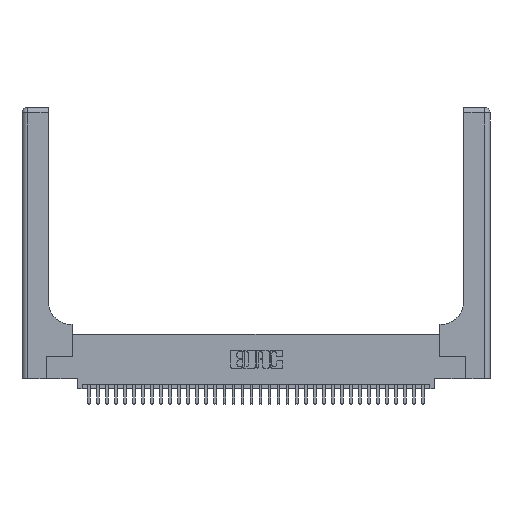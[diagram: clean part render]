
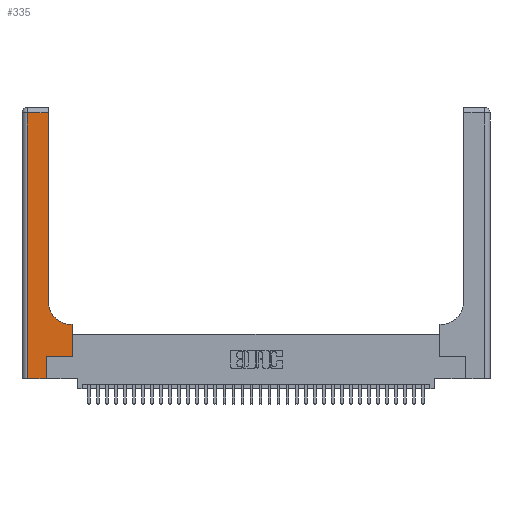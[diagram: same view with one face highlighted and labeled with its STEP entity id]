
A CAD part, top view. The second image highlights one B-rep face of the part: STEP entity #335.
In plain terms, the highlighted planar face has unit normal (0, 0, 1).
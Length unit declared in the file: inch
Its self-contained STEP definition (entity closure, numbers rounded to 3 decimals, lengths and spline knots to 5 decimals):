
#335 = ADVANCED_FACE ( 'NONE', ( #9375 ), #31112, .F. ) ;
#1353 = CARTESIAN_POINT ( 'NONE',  ( 0.269, 0.25, 0.37 ) ) ;
#1536 = DIRECTION ( 'NONE',  ( 0., 1., 0. ) ) ;
#1728 = VECTOR ( 'NONE', #20015, 39.37008 ) ;
#2449 = EDGE_CURVE ( 'NONE', #31710, #33358, #18399, .T. ) ;
#2634 = VECTOR ( 'NONE', #32224, 39.37008 ) ;
#2716 = AXIS2_PLACEMENT_3D ( 'NONE', #5078, #10599, #8089 ) ;
#4294 = DIRECTION ( 'NONE',  ( -1., 0., 0. ) ) ;
#4831 = DIRECTION ( 'NONE',  ( 1., 0., 0. ) ) ;
#5078 = CARTESIAN_POINT ( 'NONE',  ( 0.5415, 0.85, 0.37 ) ) ;
#5316 = CARTESIAN_POINT ( 'NONE',  ( 0.2915, 0.85, 0.37 ) ) ;
#5920 = LINE ( 'NONE', #24273, #15427 ) ;
#6356 = EDGE_CURVE ( 'NONE', #29898, #30478, #5920, .T. ) ;
#7204 = DIRECTION ( 'NONE',  ( 0., 0., -1. ) ) ;
#7318 = DIRECTION ( 'NONE',  ( -1., 0., 0. ) ) ;
#7488 = CARTESIAN_POINT ( 'NONE',  ( 0.269, 0.25, 0.37 ) ) ;
#8022 = CARTESIAN_POINT ( 'NONE',  ( 0.5585, 0.6, 0.37 ) ) ;
#8089 = DIRECTION ( 'NONE',  ( 1., 0., 0. ) ) ;
#8786 = AXIS2_PLACEMENT_3D ( 'NONE', #29046, #7204, #7318 ) ;
#9375 = FACE_OUTER_BOUND ( 'NONE', #27421, .T. ) ;
#10599 = DIRECTION ( 'NONE',  ( 0., 0., -1. ) ) ;
#10969 = EDGE_CURVE ( 'NONE', #17357, #12813, #31996, .T. ) ;
#10972 = DIRECTION ( 'NONE',  ( 0., 1., 0. ) ) ;
#11022 = VECTOR ( 'NONE', #26573, 39.37008 ) ;
#11787 = EDGE_CURVE ( 'NONE', #12813, #29898, #18621, .T. ) ;
#12808 = DIRECTION ( 'NONE',  ( 0., 1., 0. ) ) ;
#12813 = VERTEX_POINT ( 'NONE', #34967 ) ;
#13652 = LINE ( 'NONE', #15150, #22717 ) ;
#13897 = EDGE_CURVE ( 'NONE', #25910, #35000, #18821, .T. ) ;
#14307 = ORIENTED_EDGE ( 'NONE', *, *, #10969, .T. ) ;
#15150 = CARTESIAN_POINT ( 'NONE',  ( 0., 2.94, 0.37 ) ) ;
#15427 = VECTOR ( 'NONE', #12808, 39.37008 ) ;
#16515 = CARTESIAN_POINT ( 'NONE',  ( 0.06, 2.94, 0.37 ) ) ;
#17136 = LINE ( 'NONE', #7488, #26599 ) ;
#17357 = VERTEX_POINT ( 'NONE', #16515 ) ;
#18399 = LINE ( 'NONE', #34690, #11022 ) ;
#18621 = LINE ( 'NONE', #26267, #2634 ) ;
#18821 = LINE ( 'NONE', #30571, #29158 ) ;
#19209 = CARTESIAN_POINT ( 'NONE',  ( 0.5585, 0.25, 0.37 ) ) ;
#20015 = DIRECTION ( 'NONE',  ( 0., -1., 0. ) ) ;
#20751 = ORIENTED_EDGE ( 'NONE', *, *, #11787, .T. ) ;
#21375 = CARTESIAN_POINT ( 'NONE',  ( 0.5585, 0.25, 0.37 ) ) ;
#21390 = ORIENTED_EDGE ( 'NONE', *, *, #2449, .T. ) ;
#21697 = EDGE_CURVE ( 'NONE', #30478, #21902, #17136, .T. ) ;
#21788 = EDGE_CURVE ( 'NONE', #33358, #25910, #29222, .T. ) ;
#21902 = VERTEX_POINT ( 'NONE', #19209 ) ;
#22717 = VECTOR ( 'NONE', #4294, 39.37008 ) ;
#23096 = LINE ( 'NONE', #21375, #30869 ) ;
#23734 = CARTESIAN_POINT ( 'NONE',  ( 0.5415, 0.6, 0.37 ) ) ;
#24273 = CARTESIAN_POINT ( 'NONE',  ( 0.269, 0., 0.37 ) ) ;
#24621 = ORIENTED_EDGE ( 'NONE', *, *, #21697, .T. ) ;
#24869 = ORIENTED_EDGE ( 'NONE', *, *, #13897, .T. ) ;
#25910 = VERTEX_POINT ( 'NONE', #5316 ) ;
#26267 = CARTESIAN_POINT ( 'NONE',  ( 0., 0., 0.37 ) ) ;
#26573 = DIRECTION ( 'NONE',  ( -1., 0., 0. ) ) ;
#26599 = VECTOR ( 'NONE', #4831, 39.37008 ) ;
#27421 = EDGE_LOOP ( 'NONE', ( #24869, #27992, #14307, #20751, #32278, #24621, #33480, #21390, #33287 ) ) ;
#27992 = ORIENTED_EDGE ( 'NONE', *, *, #30461, .T. ) ;
#29046 = CARTESIAN_POINT ( 'NONE',  ( 0., 3., 0.37 ) ) ;
#29158 = VECTOR ( 'NONE', #10972, 39.37008 ) ;
#29222 = CIRCLE ( 'NONE', #2716, 0.25 ) ;
#29898 = VERTEX_POINT ( 'NONE', #34853 ) ;
#30461 = EDGE_CURVE ( 'NONE', #35000, #17357, #13652, .T. ) ;
#30478 = VERTEX_POINT ( 'NONE', #1353 ) ;
#30571 = CARTESIAN_POINT ( 'NONE',  ( 0.2915, 3., 0.37 ) ) ;
#30867 = CARTESIAN_POINT ( 'NONE',  ( 0.06, 3., 0.37 ) ) ;
#30869 = VECTOR ( 'NONE', #1536, 39.37008 ) ;
#31112 = PLANE ( 'NONE',  #8786 ) ;
#31168 = CARTESIAN_POINT ( 'NONE',  ( 0.2915, 2.94, 0.37 ) ) ;
#31710 = VERTEX_POINT ( 'NONE', #8022 ) ;
#31996 = LINE ( 'NONE', #30867, #1728 ) ;
#32224 = DIRECTION ( 'NONE',  ( 1., 0., 0. ) ) ;
#32278 = ORIENTED_EDGE ( 'NONE', *, *, #6356, .T. ) ;
#33287 = ORIENTED_EDGE ( 'NONE', *, *, #21788, .T. ) ;
#33358 = VERTEX_POINT ( 'NONE', #23734 ) ;
#33480 = ORIENTED_EDGE ( 'NONE', *, *, #34029, .T. ) ;
#34029 = EDGE_CURVE ( 'NONE', #21902, #31710, #23096, .T. ) ;
#34690 = CARTESIAN_POINT ( 'NONE',  ( 0.2915, 0.6, 0.37 ) ) ;
#34853 = CARTESIAN_POINT ( 'NONE',  ( 0.269, 0., 0.37 ) ) ;
#34967 = CARTESIAN_POINT ( 'NONE',  ( 0.06, 0., 0.37 ) ) ;
#35000 = VERTEX_POINT ( 'NONE', #31168 ) ;
